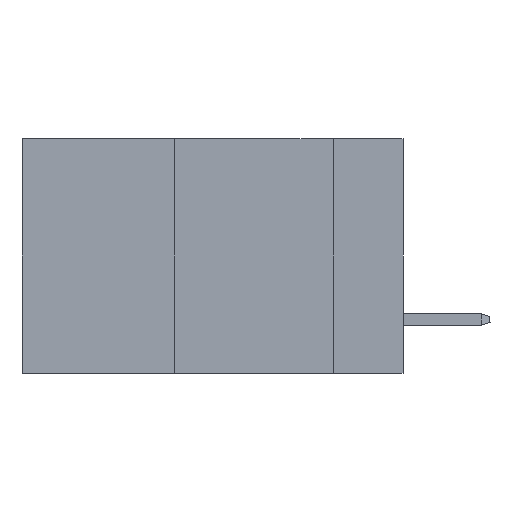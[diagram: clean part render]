
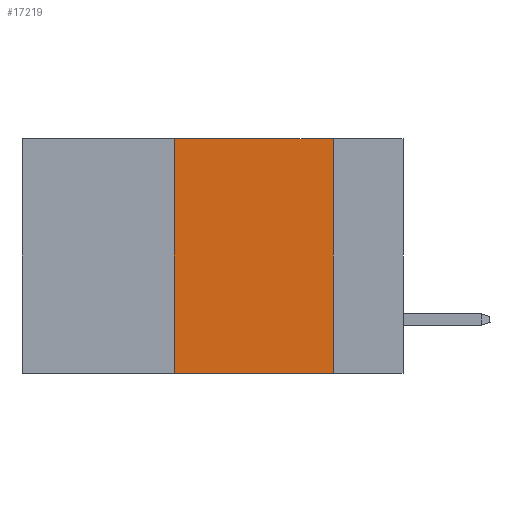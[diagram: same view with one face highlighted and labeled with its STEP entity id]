
A CAD part, left-side view. The second image highlights one B-rep face of the part: STEP entity #17219.
In plain terms, the highlighted planar face has unit normal (-1, 0, 0).
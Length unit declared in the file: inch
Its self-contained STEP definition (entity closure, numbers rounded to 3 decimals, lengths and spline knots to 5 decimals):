
#148 = PLANE ( 'NONE',  #46455 ) ;
#2298 = LINE ( 'NONE', #16665, #24445 ) ;
#2643 = ORIENTED_EDGE ( 'NONE', *, *, #41565, .F. ) ;
#3041 = EDGE_CURVE ( 'NONE', #11899, #7051, #30302, .T. ) ;
#4833 = DIRECTION ( 'NONE',  ( 0., -1., 0. ) ) ;
#5892 = DIRECTION ( 'NONE',  ( 0., 0., 1. ) ) ;
#7051 = VERTEX_POINT ( 'NONE', #23930 ) ;
#7175 = CARTESIAN_POINT ( 'NONE',  ( 0., 0.11, 0. ) ) ;
#7495 = ORIENTED_EDGE ( 'NONE', *, *, #3041, .T. ) ;
#11225 = CARTESIAN_POINT ( 'NONE',  ( 0., 0.36, -0.37 ) ) ;
#11802 = VERTEX_POINT ( 'NONE', #7175 ) ;
#11899 = VERTEX_POINT ( 'NONE', #11225 ) ;
#12660 = EDGE_CURVE ( 'NONE', #11802, #7051, #14465, .T. ) ;
#14465 = LINE ( 'NONE', #32862, #22817 ) ;
#15811 = EDGE_CURVE ( 'NONE', #11899, #36209, #2298, .T. ) ;
#16665 = CARTESIAN_POINT ( 'NONE',  ( 0., 0.36, 0. ) ) ;
#17219 = ADVANCED_FACE ( 'NONE', ( #47259 ), #148, .F. ) ;
#17582 = DIRECTION ( 'NONE',  ( 0., 0., -1. ) ) ;
#18108 = DIRECTION ( 'NONE',  ( 0., 0., -1. ) ) ;
#21812 = VECTOR ( 'NONE', #4833, 39.37008 ) ;
#22211 = CARTESIAN_POINT ( 'NONE',  ( 0., 0.6, -0.37 ) ) ;
#22817 = VECTOR ( 'NONE', #17582, 39.37008 ) ;
#23930 = CARTESIAN_POINT ( 'NONE',  ( 0., 0.11, -0.37 ) ) ;
#24445 = VECTOR ( 'NONE', #5892, 39.37008 ) ;
#25537 = CARTESIAN_POINT ( 'NONE',  ( 0., 0.6, 0. ) ) ;
#25904 = LINE ( 'NONE', #40480, #21812 ) ;
#28417 = ORIENTED_EDGE ( 'NONE', *, *, #12660, .F. ) ;
#30302 = LINE ( 'NONE', #22211, #41924 ) ;
#32862 = CARTESIAN_POINT ( 'NONE',  ( 0., 0.11, 0. ) ) ;
#34625 = CARTESIAN_POINT ( 'NONE',  ( 0., 0.36, 0. ) ) ;
#36209 = VERTEX_POINT ( 'NONE', #34625 ) ;
#36734 = DIRECTION ( 'NONE',  ( 1., 0., 0. ) ) ;
#40480 = CARTESIAN_POINT ( 'NONE',  ( 0., 0.6, 0. ) ) ;
#41057 = DIRECTION ( 'NONE',  ( 0., -1., 0. ) ) ;
#41565 = EDGE_CURVE ( 'NONE', #36209, #11802, #25904, .T. ) ;
#41924 = VECTOR ( 'NONE', #41057, 39.37008 ) ;
#45963 = EDGE_LOOP ( 'NONE', ( #28417, #2643, #46305, #7495 ) ) ;
#46305 = ORIENTED_EDGE ( 'NONE', *, *, #15811, .F. ) ;
#46455 = AXIS2_PLACEMENT_3D ( 'NONE', #25537, #36734, #18108 ) ;
#47259 = FACE_OUTER_BOUND ( 'NONE', #45963, .T. ) ;
